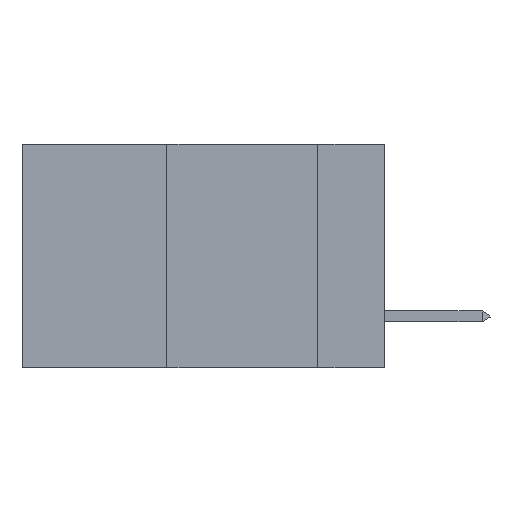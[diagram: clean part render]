
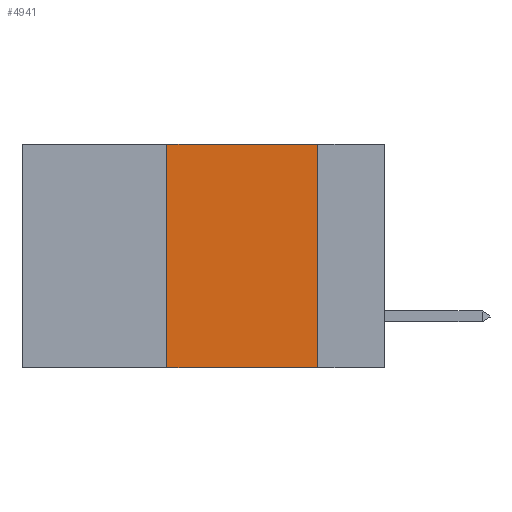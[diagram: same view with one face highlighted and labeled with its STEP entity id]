
A CAD part, left-side view. The second image highlights one B-rep face of the part: STEP entity #4941.
In plain terms, the highlighted planar face has unit normal (-1, 0, 0).
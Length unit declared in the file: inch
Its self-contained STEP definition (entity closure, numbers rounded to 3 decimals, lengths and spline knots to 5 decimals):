
#125 = VECTOR ( 'NONE', #10611, 39.37008 ) ;
#161 = DIRECTION ( 'NONE',  ( 0., 0., -1. ) ) ;
#596 = EDGE_CURVE ( 'NONE', #8133, #3630, #8791, .T. ) ;
#1516 = CARTESIAN_POINT ( 'NONE',  ( 0., 0.6, -0.37 ) ) ;
#2100 = CARTESIAN_POINT ( 'NONE',  ( 0., 0.11, 0. ) ) ;
#2417 = CARTESIAN_POINT ( 'NONE',  ( 0., 0.6, 0. ) ) ;
#2459 = DIRECTION ( 'NONE',  ( 1., 0., 0. ) ) ;
#2460 = ORIENTED_EDGE ( 'NONE', *, *, #596, .T. ) ;
#2580 = LINE ( 'NONE', #8066, #5348 ) ;
#3052 = CARTESIAN_POINT ( 'NONE',  ( 0., 0.36, -0.37 ) ) ;
#3246 = ORIENTED_EDGE ( 'NONE', *, *, #10960, .F. ) ;
#3451 = ORIENTED_EDGE ( 'NONE', *, *, #9941, .F. ) ;
#3630 = VERTEX_POINT ( 'NONE', #8328 ) ;
#3781 = AXIS2_PLACEMENT_3D ( 'NONE', #2417, #2459, #4299 ) ;
#3845 = CARTESIAN_POINT ( 'NONE',  ( 0., 0.6, 0. ) ) ;
#4165 = FACE_OUTER_BOUND ( 'NONE', #11394, .T. ) ;
#4299 = DIRECTION ( 'NONE',  ( 0., 0., -1. ) ) ;
#4941 = ADVANCED_FACE ( 'NONE', ( #4165 ), #6925, .F. ) ;
#4981 = VECTOR ( 'NONE', #10001, 39.37008 ) ;
#5348 = VECTOR ( 'NONE', #161, 39.37008 ) ;
#6608 = CARTESIAN_POINT ( 'NONE',  ( 0., 0.36, 0. ) ) ;
#6925 = PLANE ( 'NONE',  #3781 ) ;
#7207 = VERTEX_POINT ( 'NONE', #6608 ) ;
#8030 = EDGE_CURVE ( 'NONE', #9251, #3630, #2580, .T. ) ;
#8066 = CARTESIAN_POINT ( 'NONE',  ( 0., 0.11, 0. ) ) ;
#8111 = ORIENTED_EDGE ( 'NONE', *, *, #8030, .F. ) ;
#8133 = VERTEX_POINT ( 'NONE', #3052 ) ;
#8295 = LINE ( 'NONE', #3845, #4981 ) ;
#8328 = CARTESIAN_POINT ( 'NONE',  ( 0., 0.11, -0.37 ) ) ;
#8791 = LINE ( 'NONE', #1516, #10044 ) ;
#8872 = CARTESIAN_POINT ( 'NONE',  ( 0., 0.36, 0. ) ) ;
#9251 = VERTEX_POINT ( 'NONE', #2100 ) ;
#9498 = DIRECTION ( 'NONE',  ( 0., -1., 0. ) ) ;
#9917 = LINE ( 'NONE', #8872, #125 ) ;
#9941 = EDGE_CURVE ( 'NONE', #7207, #9251, #8295, .T. ) ;
#10001 = DIRECTION ( 'NONE',  ( 0., -1., 0. ) ) ;
#10044 = VECTOR ( 'NONE', #9498, 39.37008 ) ;
#10611 = DIRECTION ( 'NONE',  ( 0., 0., 1. ) ) ;
#10960 = EDGE_CURVE ( 'NONE', #8133, #7207, #9917, .T. ) ;
#11394 = EDGE_LOOP ( 'NONE', ( #8111, #3451, #3246, #2460 ) ) ;
